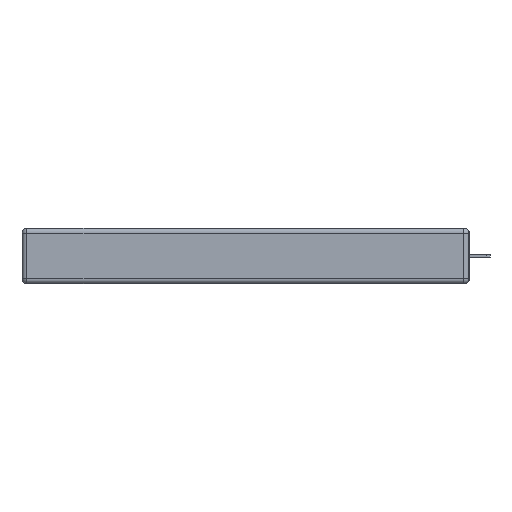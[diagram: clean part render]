
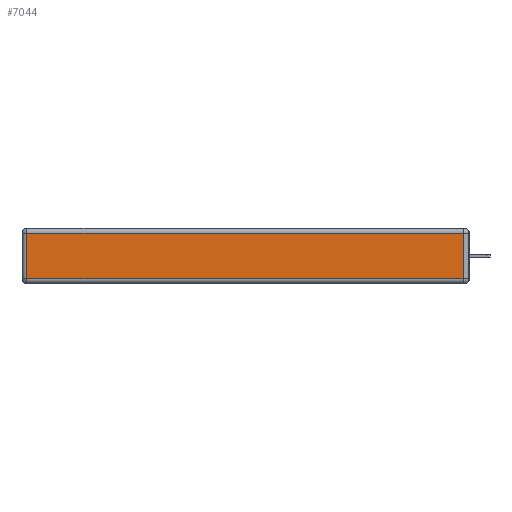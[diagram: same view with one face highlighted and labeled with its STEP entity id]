
A CAD part, left-side view. The second image highlights one B-rep face of the part: STEP entity #7044.
In plain terms, the highlighted planar face has unit normal (-1, 0, 0).
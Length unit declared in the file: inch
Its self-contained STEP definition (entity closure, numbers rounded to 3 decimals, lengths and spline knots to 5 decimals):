
#644 = EDGE_CURVE ( 'NONE', #9759, #16621, #3044, .T. ) ;
#1168 = AXIS2_PLACEMENT_3D ( 'NONE', #7301, #15439, #12878 ) ;
#1900 = VECTOR ( 'NONE', #9445, 39.37008 ) ;
#1985 = VECTOR ( 'NONE', #12528, 39.37008 ) ;
#2112 = FACE_OUTER_BOUND ( 'NONE', #10638, .T. ) ;
#3044 = LINE ( 'NONE', #7069, #1900 ) ;
#3775 = ORIENTED_EDGE ( 'NONE', *, *, #644, .T. ) ;
#3810 = EDGE_CURVE ( 'NONE', #16621, #4477, #5185, .T. ) ;
#3863 = VERTEX_POINT ( 'NONE', #17735 ) ;
#3956 = EDGE_CURVE ( 'NONE', #4477, #3863, #13653, .T. ) ;
#4477 = VERTEX_POINT ( 'NONE', #11561 ) ;
#5185 = LINE ( 'NONE', #7809, #12621 ) ;
#5274 = CARTESIAN_POINT ( 'NONE',  ( 0., 0., -0.313 ) ) ;
#5415 = CARTESIAN_POINT ( 'NONE',  ( 0., 0.03, -0.03 ) ) ;
#6217 = EDGE_CURVE ( 'NONE', #3863, #9759, #14172, .T. ) ;
#6537 = ORIENTED_EDGE ( 'NONE', *, *, #3956, .T. ) ;
#6655 = ORIENTED_EDGE ( 'NONE', *, *, #3810, .T. ) ;
#7044 = ADVANCED_FACE ( 'NONE', ( #2112 ), #7564, .T. ) ;
#7069 = CARTESIAN_POINT ( 'NONE',  ( 0., 2.75, -0.03 ) ) ;
#7301 = CARTESIAN_POINT ( 'NONE',  ( 0., 0., -0.343 ) ) ;
#7465 = CARTESIAN_POINT ( 'NONE',  ( 0., 2.72, -0.03 ) ) ;
#7564 = PLANE ( 'NONE',  #1168 ) ;
#7632 = VECTOR ( 'NONE', #9706, 39.37008 ) ;
#7809 = CARTESIAN_POINT ( 'NONE',  ( 0., 2.72, -0.343 ) ) ;
#9445 = DIRECTION ( 'NONE',  ( 0., 1., 0. ) ) ;
#9706 = DIRECTION ( 'NONE',  ( 0., -1., 0. ) ) ;
#9759 = VERTEX_POINT ( 'NONE', #5415 ) ;
#9942 = CARTESIAN_POINT ( 'NONE',  ( 0., 0.03, -0.343 ) ) ;
#10638 = EDGE_LOOP ( 'NONE', ( #6537, #13758, #3775, #6655 ) ) ;
#11561 = CARTESIAN_POINT ( 'NONE',  ( 0., 2.72, -0.313 ) ) ;
#12528 = DIRECTION ( 'NONE',  ( 0., 0., 1. ) ) ;
#12621 = VECTOR ( 'NONE', #13292, 39.37008 ) ;
#12878 = DIRECTION ( 'NONE',  ( 0., 0., 1. ) ) ;
#13292 = DIRECTION ( 'NONE',  ( 0., 0., -1. ) ) ;
#13653 = LINE ( 'NONE', #5274, #7632 ) ;
#13758 = ORIENTED_EDGE ( 'NONE', *, *, #6217, .T. ) ;
#14172 = LINE ( 'NONE', #9942, #1985 ) ;
#15439 = DIRECTION ( 'NONE',  ( -1., 0., 0. ) ) ;
#16621 = VERTEX_POINT ( 'NONE', #7465 ) ;
#17735 = CARTESIAN_POINT ( 'NONE',  ( 0., 0.03, -0.313 ) ) ;
